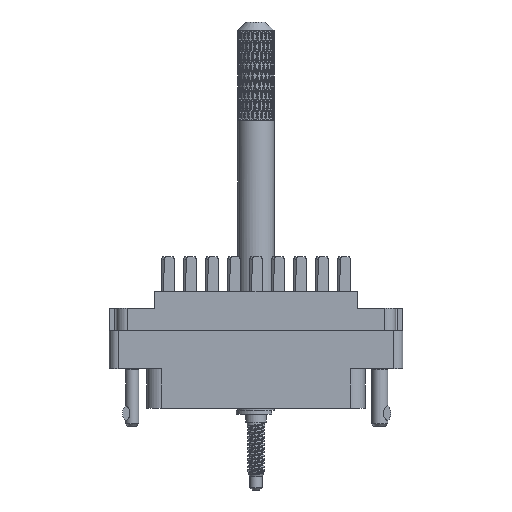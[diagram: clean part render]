
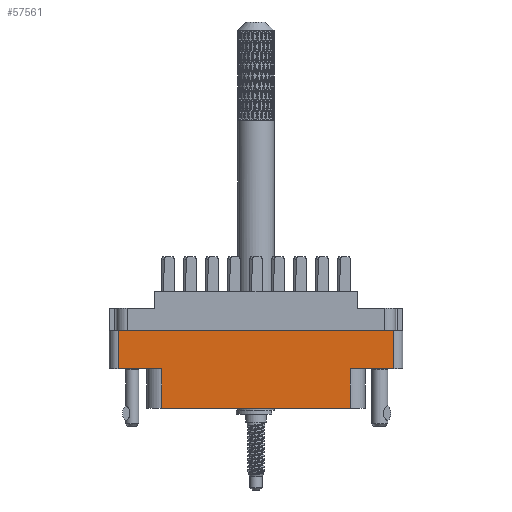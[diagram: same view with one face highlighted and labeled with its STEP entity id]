
A CAD part, front view. The second image highlights one B-rep face of the part: STEP entity #57561.
In plain terms, the highlighted planar face has unit normal (0, -1, 0).
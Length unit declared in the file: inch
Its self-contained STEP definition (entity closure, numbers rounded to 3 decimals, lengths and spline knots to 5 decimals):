
#2217 = FACE_OUTER_BOUND ( 'NONE', #71552, .T. ) ;
#2704 = AXIS2_PLACEMENT_3D ( 'NONE', #19731, #97600, #37218 ) ;
#3429 = CARTESIAN_POINT ( 'NONE',  ( 0.938, -0.438, -0.529 ) ) ;
#5241 = ORIENTED_EDGE ( 'NONE', *, *, #34193, .T. ) ;
#7444 = VERTEX_POINT ( 'NONE', #98002 ) ;
#8594 = EDGE_CURVE ( 'NONE', #80029, #52254, #106162, .T. ) ;
#10403 = CARTESIAN_POINT ( 'NONE',  ( 0.644, -0.438, -0.529 ) ) ;
#10428 = CARTESIAN_POINT ( 'NONE',  ( 0.644, -0.438, -0.529 ) ) ;
#13092 = LINE ( 'NONE', #81394, #94015 ) ;
#13410 = VERTEX_POINT ( 'NONE', #14935 ) ;
#13762 = DIRECTION ( 'NONE',  ( 0., 0., -1. ) ) ;
#14935 = CARTESIAN_POINT ( 'NONE',  ( -0.938, -0.438, -0.529 ) ) ;
#19731 = CARTESIAN_POINT ( 'NONE',  ( -0.938, -0.438, -0.798 ) ) ;
#21358 = CARTESIAN_POINT ( 'NONE',  ( -0.938, -0.438, -0.798 ) ) ;
#22192 = ORIENTED_EDGE ( 'NONE', *, *, #63945, .F. ) ;
#22646 = CARTESIAN_POINT ( 'NONE',  ( 0.938, -0.438, -0.798 ) ) ;
#23622 = DIRECTION ( 'NONE',  ( 1., 0., 0. ) ) ;
#28850 = DIRECTION ( 'NONE',  ( -1., 0., 0. ) ) ;
#32075 = CARTESIAN_POINT ( 'NONE',  ( 0., -0.438, -0.529 ) ) ;
#34193 = EDGE_CURVE ( 'NONE', #101086, #48500, #58850, .T. ) ;
#36547 = VECTOR ( 'NONE', #13762, 39.37008 ) ;
#36647 = EDGE_CURVE ( 'NONE', #13410, #50351, #40535, .T. ) ;
#37218 = DIRECTION ( 'NONE',  ( 0., 0., -1. ) ) ;
#38991 = CARTESIAN_POINT ( 'NONE',  ( -0.644, -0.438, -0.529 ) ) ;
#39200 = CARTESIAN_POINT ( 'NONE',  ( 0.644, -0.438, -0.798 ) ) ;
#39721 = CARTESIAN_POINT ( 'NONE',  ( -0.644, -0.438, -0.529 ) ) ;
#40535 = LINE ( 'NONE', #32075, #109620 ) ;
#43248 = VECTOR ( 'NONE', #83008, 39.37008 ) ;
#44437 = EDGE_CURVE ( 'NONE', #80029, #7444, #99950, .T. ) ;
#45594 = LINE ( 'NONE', #21358, #77244 ) ;
#46368 = DIRECTION ( 'NONE',  ( 1., 0., 0. ) ) ;
#48110 = ORIENTED_EDGE ( 'NONE', *, *, #75970, .F. ) ;
#48500 = VERTEX_POINT ( 'NONE', #39200 ) ;
#49461 = VECTOR ( 'NONE', #104146, 39.37008 ) ;
#50351 = VERTEX_POINT ( 'NONE', #38991 ) ;
#50371 = CARTESIAN_POINT ( 'NONE',  ( -0.938, -0.438, -0.798 ) ) ;
#52254 = VERTEX_POINT ( 'NONE', #10403 ) ;
#52372 = EDGE_CURVE ( 'NONE', #50351, #101086, #93297, .T. ) ;
#57561 = ADVANCED_FACE ( 'NONE', ( #2217 ), #95385, .T. ) ;
#58850 = LINE ( 'NONE', #50371, #68633 ) ;
#61060 = CARTESIAN_POINT ( 'NONE',  ( -0.938, -0.438, -0.268 ) ) ;
#62615 = VECTOR ( 'NONE', #28850, 39.37008 ) ;
#63945 = EDGE_CURVE ( 'NONE', #107832, #7444, #13092, .T. ) ;
#66971 = ORIENTED_EDGE ( 'NONE', *, *, #109192, .F. ) ;
#68633 = VECTOR ( 'NONE', #84826, 39.37008 ) ;
#69035 = ORIENTED_EDGE ( 'NONE', *, *, #36647, .T. ) ;
#69802 = ORIENTED_EDGE ( 'NONE', *, *, #44437, .T. ) ;
#71552 = EDGE_LOOP ( 'NONE', ( #72428, #5241, #66971, #98093, #69802, #22192, #48110, #69035 ) ) ;
#72428 = ORIENTED_EDGE ( 'NONE', *, *, #52372, .T. ) ;
#75970 = EDGE_CURVE ( 'NONE', #13410, #107832, #45594, .T. ) ;
#77244 = VECTOR ( 'NONE', #87390, 39.37008 ) ;
#80029 = VERTEX_POINT ( 'NONE', #3429 ) ;
#81394 = CARTESIAN_POINT ( 'NONE',  ( -1., -0.438, -0.268 ) ) ;
#82999 = CARTESIAN_POINT ( 'NONE',  ( 0., -0.438, -0.529 ) ) ;
#83008 = DIRECTION ( 'NONE',  ( 0., 0., 1. ) ) ;
#84826 = DIRECTION ( 'NONE',  ( 1., 0., 0. ) ) ;
#87390 = DIRECTION ( 'NONE',  ( 0., 0., 1. ) ) ;
#93297 = LINE ( 'NONE', #39721, #36547 ) ;
#94015 = VECTOR ( 'NONE', #46368, 39.37008 ) ;
#95385 = PLANE ( 'NONE',  #2704 ) ;
#97600 = DIRECTION ( 'NONE',  ( 0., -1., 0. ) ) ;
#98002 = CARTESIAN_POINT ( 'NONE',  ( 0.938, -0.438, -0.268 ) ) ;
#98093 = ORIENTED_EDGE ( 'NONE', *, *, #8594, .F. ) ;
#99950 = LINE ( 'NONE', #22646, #43248 ) ;
#101086 = VERTEX_POINT ( 'NONE', #102275 ) ;
#102275 = CARTESIAN_POINT ( 'NONE',  ( -0.644, -0.438, -0.798 ) ) ;
#103584 = LINE ( 'NONE', #10428, #49461 ) ;
#104146 = DIRECTION ( 'NONE',  ( 0., 0., -1. ) ) ;
#106162 = LINE ( 'NONE', #82999, #62615 ) ;
#107832 = VERTEX_POINT ( 'NONE', #61060 ) ;
#109192 = EDGE_CURVE ( 'NONE', #52254, #48500, #103584, .T. ) ;
#109620 = VECTOR ( 'NONE', #23622, 39.37008 ) ;
